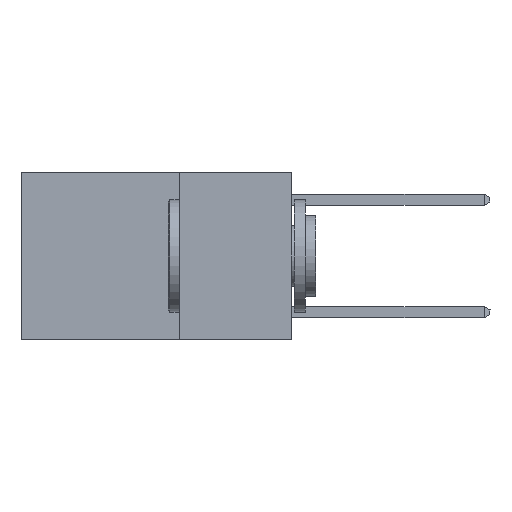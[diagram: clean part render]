
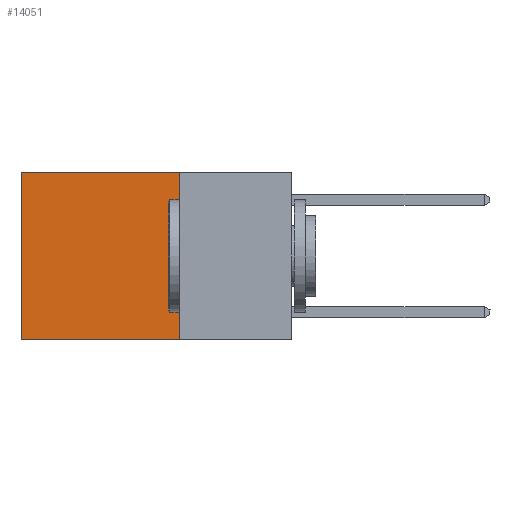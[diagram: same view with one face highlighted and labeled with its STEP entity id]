
A CAD part, left-side view. The second image highlights one B-rep face of the part: STEP entity #14051.
In plain terms, the highlighted planar face has unit normal (-1, 0, 0).
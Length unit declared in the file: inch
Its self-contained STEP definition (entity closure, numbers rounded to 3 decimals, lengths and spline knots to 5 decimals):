
#482 = VECTOR ( 'NONE', #4856, 39.37008 ) ;
#1406 = VERTEX_POINT ( 'NONE', #11194 ) ;
#1619 = VECTOR ( 'NONE', #24968, 39.37008 ) ;
#1886 = EDGE_CURVE ( 'NONE', #1406, #23928, #17256, .T. ) ;
#4484 = CARTESIAN_POINT ( 'NONE',  ( 0.2625, 0.6, 0. ) ) ;
#4854 = CARTESIAN_POINT ( 'NONE',  ( 0.2625, 0.25, 0. ) ) ;
#4856 = DIRECTION ( 'NONE',  ( 0., 0., -1. ) ) ;
#5458 = CARTESIAN_POINT ( 'NONE',  ( 0.2625, 0.25, -0.37 ) ) ;
#6537 = DIRECTION ( 'NONE',  ( 0., 0., -1. ) ) ;
#7049 = FACE_OUTER_BOUND ( 'NONE', #19240, .T. ) ;
#7069 = LINE ( 'NONE', #19346, #1619 ) ;
#7448 = VERTEX_POINT ( 'NONE', #8309 ) ;
#8309 = CARTESIAN_POINT ( 'NONE',  ( 0.2625, 0.6, -0.37 ) ) ;
#10948 = DIRECTION ( 'NONE',  ( 0., 0., -1. ) ) ;
#11194 = CARTESIAN_POINT ( 'NONE',  ( 0.2625, 0.25, 0. ) ) ;
#11643 = ORIENTED_EDGE ( 'NONE', *, *, #23615, .T. ) ;
#11885 = EDGE_CURVE ( 'NONE', #23928, #7448, #18248, .T. ) ;
#13080 = VECTOR ( 'NONE', #16111, 39.37008 ) ;
#13633 = EDGE_CURVE ( 'NONE', #1406, #18072, #7069, .T. ) ;
#14051 = ADVANCED_FACE ( 'NONE', ( #7049 ), #20567, .F. ) ;
#14314 = ORIENTED_EDGE ( 'NONE', *, *, #1886, .F. ) ;
#15481 = CARTESIAN_POINT ( 'NONE',  ( 0.2625, 0.6, 0. ) ) ;
#15505 = ORIENTED_EDGE ( 'NONE', *, *, #13633, .T. ) ;
#15547 = AXIS2_PLACEMENT_3D ( 'NONE', #20649, #22555, #10948 ) ;
#16111 = DIRECTION ( 'NONE',  ( 0., 1., 0. ) ) ;
#16949 = ORIENTED_EDGE ( 'NONE', *, *, #11885, .F. ) ;
#16994 = VECTOR ( 'NONE', #6537, 39.37008 ) ;
#17256 = LINE ( 'NONE', #4854, #482 ) ;
#17604 = LINE ( 'NONE', #4484, #16994 ) ;
#18072 = VERTEX_POINT ( 'NONE', #15481 ) ;
#18248 = LINE ( 'NONE', #19908, #13080 ) ;
#19240 = EDGE_LOOP ( 'NONE', ( #11643, #16949, #14314, #15505 ) ) ;
#19346 = CARTESIAN_POINT ( 'NONE',  ( 0.2625, 0.25, 0. ) ) ;
#19908 = CARTESIAN_POINT ( 'NONE',  ( 0.2625, 0.25, -0.37 ) ) ;
#20567 = PLANE ( 'NONE',  #15547 ) ;
#20649 = CARTESIAN_POINT ( 'NONE',  ( 0.2625, 0.25, 0. ) ) ;
#22555 = DIRECTION ( 'NONE',  ( 1., 0., 0. ) ) ;
#23615 = EDGE_CURVE ( 'NONE', #18072, #7448, #17604, .T. ) ;
#23928 = VERTEX_POINT ( 'NONE', #5458 ) ;
#24968 = DIRECTION ( 'NONE',  ( 0., 1., 0. ) ) ;
